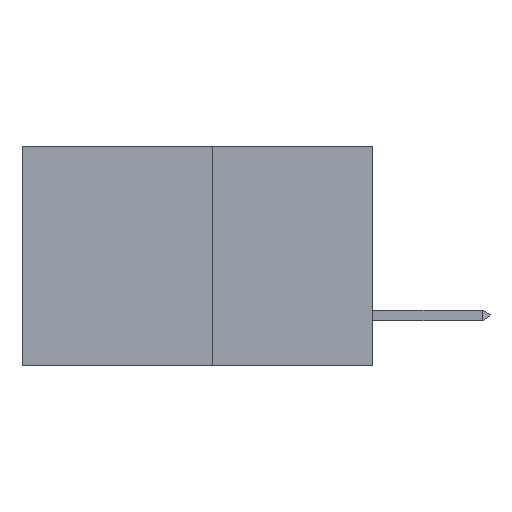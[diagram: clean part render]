
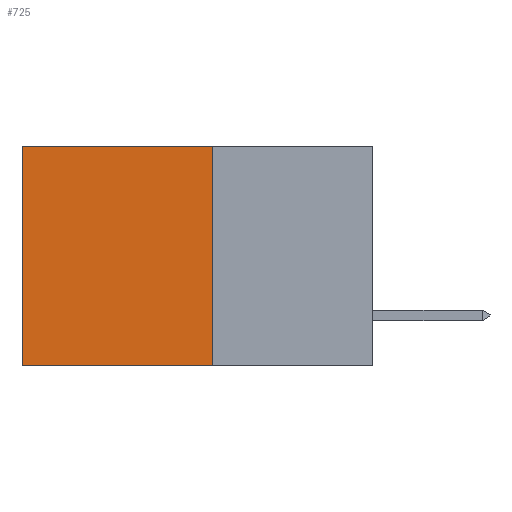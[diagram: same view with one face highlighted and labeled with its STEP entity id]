
A CAD part, left-side view. The second image highlights one B-rep face of the part: STEP entity #725.
In plain terms, the highlighted planar face has unit normal (-1, 0, 0).
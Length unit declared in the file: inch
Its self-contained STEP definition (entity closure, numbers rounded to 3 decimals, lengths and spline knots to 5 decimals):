
#263 = DIRECTION ( 'NONE',  ( 0., 0., -1. ) ) ;
#694 = VECTOR ( 'NONE', #263, 39.37008 ) ;
#725 = ADVANCED_FACE ( 'NONE', ( #21356 ), #16484, .F. ) ;
#1885 = CARTESIAN_POINT ( 'NONE',  ( 0.277, 0.27, -0.37 ) ) ;
#2055 = CARTESIAN_POINT ( 'NONE',  ( 0.277, 0.59, 0. ) ) ;
#2984 = EDGE_CURVE ( 'NONE', #13908, #4278, #9277, .T. ) ;
#3457 = EDGE_CURVE ( 'NONE', #14509, #11604, #17596, .T. ) ;
#3767 = DIRECTION ( 'NONE',  ( 0., 1., 0. ) ) ;
#3861 = DIRECTION ( 'NONE',  ( 0., 0., -1. ) ) ;
#4268 = VECTOR ( 'NONE', #3767, 39.37008 ) ;
#4278 = VERTEX_POINT ( 'NONE', #9202 ) ;
#4356 = CARTESIAN_POINT ( 'NONE',  ( 0.277, 0.27, -0.37 ) ) ;
#5664 = EDGE_LOOP ( 'NONE', ( #9322, #15581, #11056, #5969 ) ) ;
#5969 = ORIENTED_EDGE ( 'NONE', *, *, #3457, .T. ) ;
#7203 = CARTESIAN_POINT ( 'NONE',  ( 0.277, 0.59, -0.37 ) ) ;
#7499 = CARTESIAN_POINT ( 'NONE',  ( 0.277, 0.27, -0.37 ) ) ;
#9202 = CARTESIAN_POINT ( 'NONE',  ( 0.277, 0.59, -0.37 ) ) ;
#9277 = LINE ( 'NONE', #4356, #4268 ) ;
#9322 = ORIENTED_EDGE ( 'NONE', *, *, #14266, .T. ) ;
#9584 = CARTESIAN_POINT ( 'NONE',  ( 0.277, 0.27, 0. ) ) ;
#9928 = DIRECTION ( 'NONE',  ( 0., 0., -1. ) ) ;
#11056 = ORIENTED_EDGE ( 'NONE', *, *, #14085, .F. ) ;
#11117 = CARTESIAN_POINT ( 'NONE',  ( 0.277, 0.27, -0.37 ) ) ;
#11604 = VERTEX_POINT ( 'NONE', #2055 ) ;
#12236 = AXIS2_PLACEMENT_3D ( 'NONE', #7499, #13733, #9928 ) ;
#13733 = DIRECTION ( 'NONE',  ( 1., 0., 0. ) ) ;
#13908 = VERTEX_POINT ( 'NONE', #11117 ) ;
#14000 = LINE ( 'NONE', #1885, #694 ) ;
#14085 = EDGE_CURVE ( 'NONE', #14509, #13908, #14000, .T. ) ;
#14266 = EDGE_CURVE ( 'NONE', #11604, #4278, #15266, .T. ) ;
#14509 = VERTEX_POINT ( 'NONE', #9584 ) ;
#15266 = LINE ( 'NONE', #7203, #19181 ) ;
#15581 = ORIENTED_EDGE ( 'NONE', *, *, #2984, .F. ) ;
#16484 = PLANE ( 'NONE',  #12236 ) ;
#16547 = VECTOR ( 'NONE', #18635, 39.37008 ) ;
#17596 = LINE ( 'NONE', #18154, #16547 ) ;
#18154 = CARTESIAN_POINT ( 'NONE',  ( 0.277, 0.27, 0. ) ) ;
#18635 = DIRECTION ( 'NONE',  ( 0., 1., 0. ) ) ;
#19181 = VECTOR ( 'NONE', #3861, 39.37008 ) ;
#21356 = FACE_OUTER_BOUND ( 'NONE', #5664, .T. ) ;
